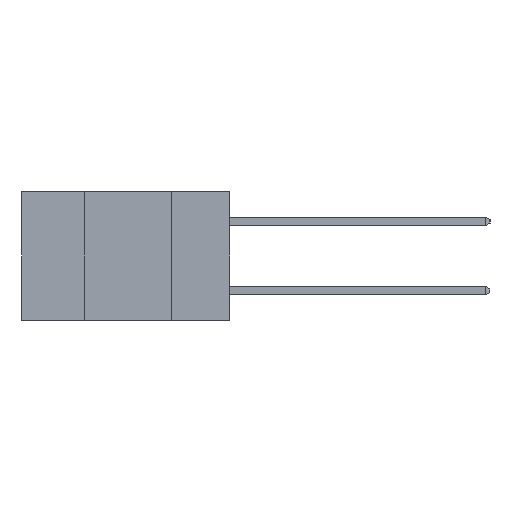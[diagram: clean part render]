
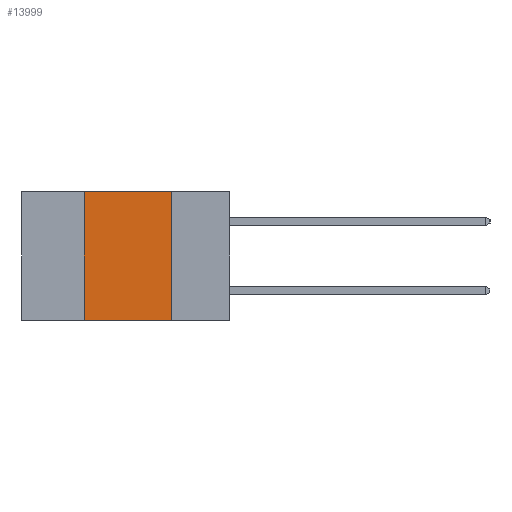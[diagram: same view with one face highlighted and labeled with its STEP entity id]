
A CAD part, left-side view. The second image highlights one B-rep face of the part: STEP entity #13999.
In plain terms, the highlighted planar face has unit normal (-1, 0, 0).
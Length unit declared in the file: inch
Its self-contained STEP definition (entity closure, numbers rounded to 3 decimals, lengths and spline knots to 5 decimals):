
#65 = CARTESIAN_POINT ( 'NONE',  ( 0., 0.17, -0.37 ) ) ;
#317 = EDGE_CURVE ( 'NONE', #11566, #8742, #16447, .T. ) ;
#1588 = CARTESIAN_POINT ( 'NONE',  ( 0., 0.17, 0. ) ) ;
#1636 = EDGE_CURVE ( 'NONE', #8742, #5330, #13532, .T. ) ;
#2098 = ORIENTED_EDGE ( 'NONE', *, *, #22155, .T. ) ;
#4157 = ORIENTED_EDGE ( 'NONE', *, *, #23388, .F. ) ;
#4515 = VECTOR ( 'NONE', #18860, 39.37008 ) ;
#5109 = LINE ( 'NONE', #7710, #4515 ) ;
#5330 = VERTEX_POINT ( 'NONE', #6760 ) ;
#6184 = CARTESIAN_POINT ( 'NONE',  ( 0., 0.42, 0. ) ) ;
#6245 = ORIENTED_EDGE ( 'NONE', *, *, #317, .F. ) ;
#6500 = AXIS2_PLACEMENT_3D ( 'NONE', #22100, #10986, #23959 ) ;
#6760 = CARTESIAN_POINT ( 'NONE',  ( 0., 0.17, -0.37 ) ) ;
#7108 = VECTOR ( 'NONE', #14004, 39.37008 ) ;
#7231 = PLANE ( 'NONE',  #6500 ) ;
#7710 = CARTESIAN_POINT ( 'NONE',  ( 0., 0.6, -0.37 ) ) ;
#7744 = CARTESIAN_POINT ( 'NONE',  ( 0., 0.42, -0.37 ) ) ;
#7937 = VECTOR ( 'NONE', #19737, 39.37008 ) ;
#8742 = VERTEX_POINT ( 'NONE', #1588 ) ;
#9619 = DIRECTION ( 'NONE',  ( 0., 0., 1. ) ) ;
#10986 = DIRECTION ( 'NONE',  ( 1., 0., 0. ) ) ;
#11073 = EDGE_LOOP ( 'NONE', ( #19316, #6245, #4157, #2098 ) ) ;
#11451 = VERTEX_POINT ( 'NONE', #13316 ) ;
#11566 = VERTEX_POINT ( 'NONE', #6184 ) ;
#13316 = CARTESIAN_POINT ( 'NONE',  ( 0., 0.42, -0.37 ) ) ;
#13532 = LINE ( 'NONE', #65, #7937 ) ;
#13999 = ADVANCED_FACE ( 'NONE', ( #22556 ), #7231, .F. ) ;
#14004 = DIRECTION ( 'NONE',  ( 0., -1., 0. ) ) ;
#16447 = LINE ( 'NONE', #17289, #7108 ) ;
#16765 = VECTOR ( 'NONE', #9619, 39.37008 ) ;
#17289 = CARTESIAN_POINT ( 'NONE',  ( 0., 0.6, 0. ) ) ;
#17331 = LINE ( 'NONE', #7744, #16765 ) ;
#18860 = DIRECTION ( 'NONE',  ( 0., -1., 0. ) ) ;
#19316 = ORIENTED_EDGE ( 'NONE', *, *, #1636, .F. ) ;
#19737 = DIRECTION ( 'NONE',  ( 0., 0., -1. ) ) ;
#22100 = CARTESIAN_POINT ( 'NONE',  ( 0., 0.6, 0. ) ) ;
#22155 = EDGE_CURVE ( 'NONE', #11451, #5330, #5109, .T. ) ;
#22556 = FACE_OUTER_BOUND ( 'NONE', #11073, .T. ) ;
#23388 = EDGE_CURVE ( 'NONE', #11451, #11566, #17331, .T. ) ;
#23959 = DIRECTION ( 'NONE',  ( 0., 0., -1. ) ) ;
